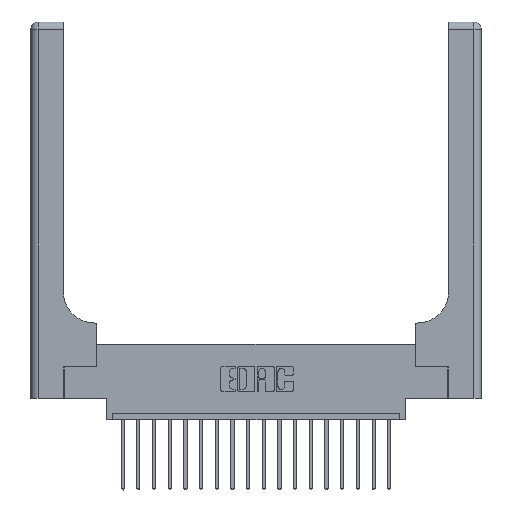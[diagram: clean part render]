
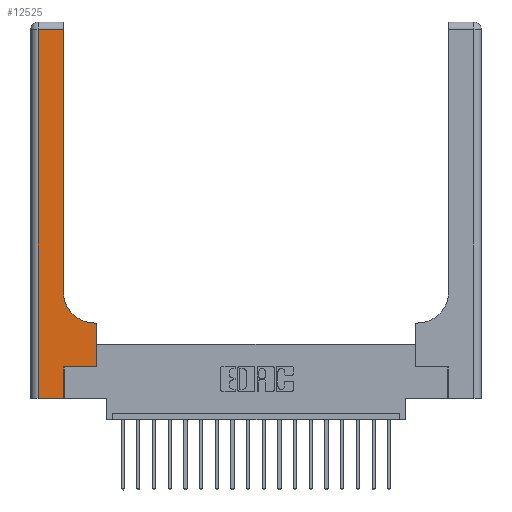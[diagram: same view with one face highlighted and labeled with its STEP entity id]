
A CAD part, top view. The second image highlights one B-rep face of the part: STEP entity #12525.
In plain terms, the highlighted planar face has unit normal (0, 0, 1).
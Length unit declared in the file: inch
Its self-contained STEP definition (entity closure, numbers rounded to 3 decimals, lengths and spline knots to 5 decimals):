
#121 = FACE_OUTER_BOUND ( 'NONE', #14272, .T. ) ;
#358 = EDGE_CURVE ( 'NONE', #4197, #12014, #12408, .T. ) ;
#650 = LINE ( 'NONE', #6129, #18079 ) ;
#1357 = LINE ( 'NONE', #13167, #8023 ) ;
#1422 = CARTESIAN_POINT ( 'NONE',  ( 0.51, 0.6, 0.37 ) ) ;
#2461 = EDGE_CURVE ( 'NONE', #12014, #6266, #650, .T. ) ;
#2565 = VERTEX_POINT ( 'NONE', #13713 ) ;
#2775 = CARTESIAN_POINT ( 'NONE',  ( 0., 2.94, 0.37 ) ) ;
#2990 = EDGE_CURVE ( 'NONE', #7939, #4197, #16879, .T. ) ;
#3486 = VECTOR ( 'NONE', #7135, 39.37008 ) ;
#3804 = CARTESIAN_POINT ( 'NONE',  ( 0.265, 0., 0.37 ) ) ;
#3805 = CARTESIAN_POINT ( 'NONE',  ( 0., 0., 0.37 ) ) ;
#4114 = ORIENTED_EDGE ( 'NONE', *, *, #2990, .T. ) ;
#4197 = VERTEX_POINT ( 'NONE', #4595 ) ;
#4437 = VECTOR ( 'NONE', #7889, 39.37008 ) ;
#4595 = CARTESIAN_POINT ( 'NONE',  ( 0.06, 0., 0.37 ) ) ;
#5027 = VECTOR ( 'NONE', #6665, 39.37008 ) ;
#6129 = CARTESIAN_POINT ( 'NONE',  ( 0.265, 0., 0.37 ) ) ;
#6266 = VERTEX_POINT ( 'NONE', #9984 ) ;
#6337 = CIRCLE ( 'NONE', #10080, 0.25 ) ;
#6507 = VERTEX_POINT ( 'NONE', #14749 ) ;
#6665 = DIRECTION ( 'NONE',  ( 1., 0., 0. ) ) ;
#6829 = VECTOR ( 'NONE', #9006, 39.37008 ) ;
#7041 = CARTESIAN_POINT ( 'NONE',  ( 0., 3., 0.37 ) ) ;
#7135 = DIRECTION ( 'NONE',  ( 0., -1., 0. ) ) ;
#7157 = ORIENTED_EDGE ( 'NONE', *, *, #19422, .T. ) ;
#7629 = ORIENTED_EDGE ( 'NONE', *, *, #358, .T. ) ;
#7889 = DIRECTION ( 'NONE',  ( 0., 1., 0. ) ) ;
#7913 = ORIENTED_EDGE ( 'NONE', *, *, #13424, .T. ) ;
#7939 = VERTEX_POINT ( 'NONE', #12613 ) ;
#8023 = VECTOR ( 'NONE', #8665, 39.37008 ) ;
#8665 = DIRECTION ( 'NONE',  ( 0., 1., 0. ) ) ;
#8731 = LINE ( 'NONE', #8866, #6829 ) ;
#8769 = CARTESIAN_POINT ( 'NONE',  ( 0.51, 0.85, 0.37 ) ) ;
#8866 = CARTESIAN_POINT ( 'NONE',  ( 0.26, 0.6, 0.37 ) ) ;
#9006 = DIRECTION ( 'NONE',  ( -1., 0., 0. ) ) ;
#9291 = DIRECTION ( 'NONE',  ( 1., 0., 0. ) ) ;
#9471 = ORIENTED_EDGE ( 'NONE', *, *, #11137, .T. ) ;
#9984 = CARTESIAN_POINT ( 'NONE',  ( 0.265, 0.25, 0.37 ) ) ;
#9989 = VERTEX_POINT ( 'NONE', #17612 ) ;
#10080 = AXIS2_PLACEMENT_3D ( 'NONE', #8769, #16470, #12097 ) ;
#10394 = VECTOR ( 'NONE', #13445, 39.37008 ) ;
#10608 = LINE ( 'NONE', #10895, #4437 ) ;
#10895 = CARTESIAN_POINT ( 'NONE',  ( 0.528, 0.25, 0.37 ) ) ;
#11137 = EDGE_CURVE ( 'NONE', #6507, #9989, #1357, .T. ) ;
#11242 = VECTOR ( 'NONE', #9291, 39.37008 ) ;
#11518 = ORIENTED_EDGE ( 'NONE', *, *, #14794, .T. ) ;
#11934 = VERTEX_POINT ( 'NONE', #15535 ) ;
#12014 = VERTEX_POINT ( 'NONE', #3804 ) ;
#12097 = DIRECTION ( 'NONE',  ( 1., 0., 0. ) ) ;
#12408 = LINE ( 'NONE', #3805, #5027 ) ;
#12455 = LINE ( 'NONE', #17019, #11242 ) ;
#12525 = ADVANCED_FACE ( 'NONE', ( #121 ), #14816, .F. ) ;
#12613 = CARTESIAN_POINT ( 'NONE',  ( 0.06, 2.94, 0.37 ) ) ;
#13167 = CARTESIAN_POINT ( 'NONE',  ( 0.26, 3., 0.37 ) ) ;
#13293 = CARTESIAN_POINT ( 'NONE',  ( 0.06, 3., 0.37 ) ) ;
#13397 = AXIS2_PLACEMENT_3D ( 'NONE', #7041, #19350, #17902 ) ;
#13424 = EDGE_CURVE ( 'NONE', #2565, #11934, #10608, .T. ) ;
#13445 = DIRECTION ( 'NONE',  ( -1., 0., 0. ) ) ;
#13713 = CARTESIAN_POINT ( 'NONE',  ( 0.528, 0.25, 0.37 ) ) ;
#13927 = EDGE_CURVE ( 'NONE', #9989, #7939, #14498, .T. ) ;
#14272 = EDGE_LOOP ( 'NONE', ( #9471, #17372, #4114, #7629, #15790, #19635, #7913, #7157, #11518 ) ) ;
#14361 = DIRECTION ( 'NONE',  ( 0., 1., 0. ) ) ;
#14498 = LINE ( 'NONE', #2775, #10394 ) ;
#14749 = CARTESIAN_POINT ( 'NONE',  ( 0.26, 0.85, 0.37 ) ) ;
#14794 = EDGE_CURVE ( 'NONE', #16814, #6507, #6337, .T. ) ;
#14816 = PLANE ( 'NONE',  #13397 ) ;
#15535 = CARTESIAN_POINT ( 'NONE',  ( 0.528, 0.6, 0.37 ) ) ;
#15790 = ORIENTED_EDGE ( 'NONE', *, *, #2461, .T. ) ;
#16453 = EDGE_CURVE ( 'NONE', #6266, #2565, #12455, .T. ) ;
#16470 = DIRECTION ( 'NONE',  ( 0., 0., -1. ) ) ;
#16814 = VERTEX_POINT ( 'NONE', #1422 ) ;
#16879 = LINE ( 'NONE', #13293, #3486 ) ;
#17019 = CARTESIAN_POINT ( 'NONE',  ( 0.265, 0.25, 0.37 ) ) ;
#17372 = ORIENTED_EDGE ( 'NONE', *, *, #13927, .T. ) ;
#17612 = CARTESIAN_POINT ( 'NONE',  ( 0.26, 2.94, 0.37 ) ) ;
#17902 = DIRECTION ( 'NONE',  ( -1., 0., 0. ) ) ;
#18079 = VECTOR ( 'NONE', #14361, 39.37008 ) ;
#19350 = DIRECTION ( 'NONE',  ( 0., 0., -1. ) ) ;
#19422 = EDGE_CURVE ( 'NONE', #11934, #16814, #8731, .T. ) ;
#19635 = ORIENTED_EDGE ( 'NONE', *, *, #16453, .T. ) ;
